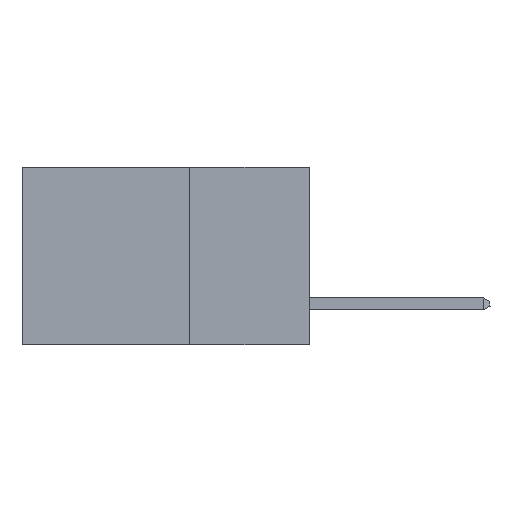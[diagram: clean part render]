
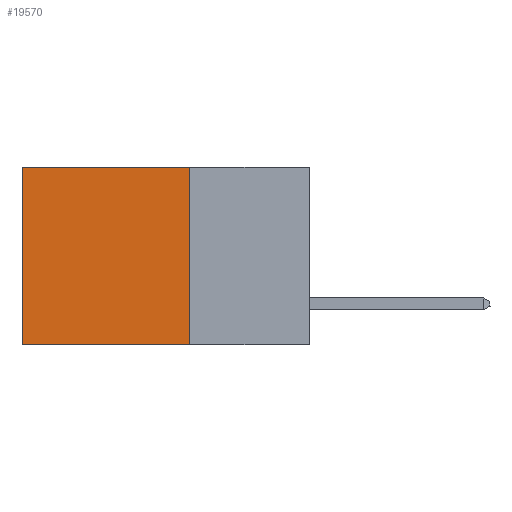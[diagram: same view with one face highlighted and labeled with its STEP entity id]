
A CAD part, left-side view. The second image highlights one B-rep face of the part: STEP entity #19570.
In plain terms, the highlighted planar face has unit normal (-1, 0, 0).
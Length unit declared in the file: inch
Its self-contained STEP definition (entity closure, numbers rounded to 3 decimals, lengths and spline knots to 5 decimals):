
#1447 = CARTESIAN_POINT ( 'NONE',  ( 0.2875, 0.25, 0. ) ) ;
#2065 = ORIENTED_EDGE ( 'NONE', *, *, #8101, .T. ) ;
#2071 = ORIENTED_EDGE ( 'NONE', *, *, #12685, .F. ) ;
#3082 = FACE_OUTER_BOUND ( 'NONE', #16054, .T. ) ;
#4450 = ORIENTED_EDGE ( 'NONE', *, *, #16698, .F. ) ;
#4840 = CARTESIAN_POINT ( 'NONE',  ( 0.2875, 0.6, 0. ) ) ;
#5087 = LINE ( 'NONE', #4840, #12771 ) ;
#5256 = CARTESIAN_POINT ( 'NONE',  ( 0.2875, 0.25, 0. ) ) ;
#5295 = VECTOR ( 'NONE', #8931, 39.37008 ) ;
#5945 = CARTESIAN_POINT ( 'NONE',  ( 0.2875, 0.25, -0.37 ) ) ;
#6881 = DIRECTION ( 'NONE',  ( 0., 0., -1. ) ) ;
#8101 = EDGE_CURVE ( 'NONE', #12954, #20108, #17855, .T. ) ;
#8212 = LINE ( 'NONE', #19180, #13079 ) ;
#8931 = DIRECTION ( 'NONE',  ( 0., 1., 0. ) ) ;
#10687 = VERTEX_POINT ( 'NONE', #20431 ) ;
#11751 = ORIENTED_EDGE ( 'NONE', *, *, #19218, .T. ) ;
#12685 = EDGE_CURVE ( 'NONE', #21711, #10687, #8212, .T. ) ;
#12771 = VECTOR ( 'NONE', #19567, 39.37008 ) ;
#12954 = VERTEX_POINT ( 'NONE', #13578 ) ;
#13079 = VECTOR ( 'NONE', #22900, 39.37008 ) ;
#13578 = CARTESIAN_POINT ( 'NONE',  ( 0.2875, 0.25, 0. ) ) ;
#15851 = DIRECTION ( 'NONE',  ( 0., 0., -1. ) ) ;
#16054 = EDGE_LOOP ( 'NONE', ( #11751, #2071, #4450, #2065 ) ) ;
#16698 = EDGE_CURVE ( 'NONE', #12954, #21711, #16859, .T. ) ;
#16859 = LINE ( 'NONE', #1447, #17728 ) ;
#17728 = VECTOR ( 'NONE', #15851, 39.37008 ) ;
#17855 = LINE ( 'NONE', #5256, #5295 ) ;
#19180 = CARTESIAN_POINT ( 'NONE',  ( 0.2875, 0.25, -0.37 ) ) ;
#19218 = EDGE_CURVE ( 'NONE', #20108, #10687, #5087, .T. ) ;
#19567 = DIRECTION ( 'NONE',  ( 0., 0., -1. ) ) ;
#19570 = ADVANCED_FACE ( 'NONE', ( #3082 ), #22004, .F. ) ;
#20108 = VERTEX_POINT ( 'NONE', #21426 ) ;
#20431 = CARTESIAN_POINT ( 'NONE',  ( 0.2875, 0.6, -0.37 ) ) ;
#20498 = CARTESIAN_POINT ( 'NONE',  ( 0.2875, 0.25, 0. ) ) ;
#21426 = CARTESIAN_POINT ( 'NONE',  ( 0.2875, 0.6, 0. ) ) ;
#21711 = VERTEX_POINT ( 'NONE', #5945 ) ;
#22004 = PLANE ( 'NONE',  #22185 ) ;
#22132 = DIRECTION ( 'NONE',  ( 1., 0., 0. ) ) ;
#22185 = AXIS2_PLACEMENT_3D ( 'NONE', #20498, #22132, #6881 ) ;
#22900 = DIRECTION ( 'NONE',  ( 0., 1., 0. ) ) ;
